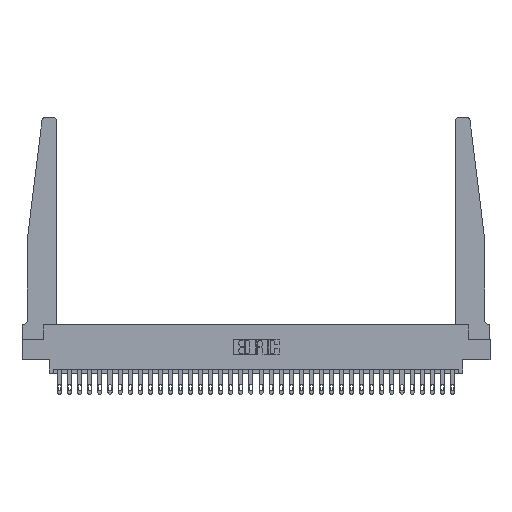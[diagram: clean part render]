
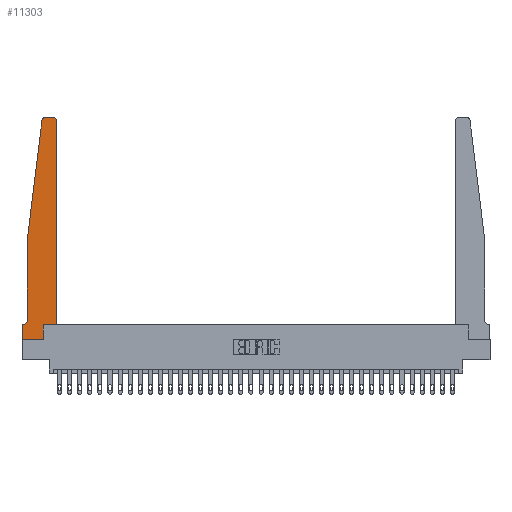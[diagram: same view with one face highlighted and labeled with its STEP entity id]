
A CAD part, top view. The second image highlights one B-rep face of the part: STEP entity #11303.
In plain terms, the highlighted planar face has unit normal (0, 0, 1).
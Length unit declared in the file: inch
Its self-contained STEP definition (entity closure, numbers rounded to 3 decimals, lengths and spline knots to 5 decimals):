
#123 = EDGE_CURVE ( 'NONE', #7158, #9645, #1898, .T. ) ;
#701 = LINE ( 'NONE', #27002, #2936 ) ;
#1346 = VECTOR ( 'NONE', #9634, 39.37008 ) ;
#1495 = VERTEX_POINT ( 'NONE', #11443 ) ;
#1792 = DIRECTION ( 'NONE',  ( -1., 0., 0. ) ) ;
#1898 = CIRCLE ( 'NONE', #8048, 0.03 ) ;
#1957 = EDGE_CURVE ( 'NONE', #8215, #24867, #27347, .T. ) ;
#2652 = FACE_OUTER_BOUND ( 'NONE', #3801, .T. ) ;
#2743 = LINE ( 'NONE', #31608, #1346 ) ;
#2936 = VECTOR ( 'NONE', #10459, 39.37008 ) ;
#3801 = EDGE_LOOP ( 'NONE', ( #6980, #9126, #20658, #7525, #21040, #28961, #9816, #30972, #6041, #6611, #29321, #30277 ) ) ;
#4433 = CARTESIAN_POINT ( 'NONE',  ( 0.065, 1.25, 0.37 ) ) ;
#4460 = AXIS2_PLACEMENT_3D ( 'NONE', #30757, #18735, #13747 ) ;
#4726 = CARTESIAN_POINT ( 'NONE',  ( 0.27653, 2.75, 0.37 ) ) ;
#4732 = VERTEX_POINT ( 'NONE', #18431 ) ;
#5006 = VECTOR ( 'NONE', #24131, 39.37008 ) ;
#5258 = CARTESIAN_POINT ( 'NONE',  ( 0.395, 2.75, 0.37 ) ) ;
#5487 = LINE ( 'NONE', #7716, #8465 ) ;
#5634 = CARTESIAN_POINT ( 'NONE',  ( 0.2605, 0., 0.37 ) ) ;
#6041 = ORIENTED_EDGE ( 'NONE', *, *, #28409, .T. ) ;
#6611 = ORIENTED_EDGE ( 'NONE', *, *, #25620, .T. ) ;
#6639 = CARTESIAN_POINT ( 'NONE',  ( 0.27653, 2.72, 0.37 ) ) ;
#6980 = ORIENTED_EDGE ( 'NONE', *, *, #19520, .T. ) ;
#7150 = CARTESIAN_POINT ( 'NONE',  ( 0., 0.1875, 0.37 ) ) ;
#7158 = VERTEX_POINT ( 'NONE', #28090 ) ;
#7253 = VERTEX_POINT ( 'NONE', #18479 ) ;
#7525 = ORIENTED_EDGE ( 'NONE', *, *, #24186, .T. ) ;
#7612 = CARTESIAN_POINT ( 'NONE',  ( 0.2605, 0.18, 0.37 ) ) ;
#7716 = CARTESIAN_POINT ( 'NONE',  ( 0.425, 0.18, 0.37 ) ) ;
#8041 = CARTESIAN_POINT ( 'NONE',  ( 0.065, 1.25, 0.37 ) ) ;
#8048 = AXIS2_PLACEMENT_3D ( 'NONE', #25898, #28929, #28639 ) ;
#8215 = VERTEX_POINT ( 'NONE', #4726 ) ;
#8465 = VECTOR ( 'NONE', #10102, 39.37008 ) ;
#8737 = CARTESIAN_POINT ( 'NONE',  ( 0.24675, 2.72367, 0.37 ) ) ;
#8828 = CARTESIAN_POINT ( 'NONE',  ( 0.425, 0.18, 0.37 ) ) ;
#8996 = LINE ( 'NONE', #13953, #21807 ) ;
#9024 = AXIS2_PLACEMENT_3D ( 'NONE', #7150, #16941, #9701 ) ;
#9095 = VERTEX_POINT ( 'NONE', #30935 ) ;
#9126 = ORIENTED_EDGE ( 'NONE', *, *, #1957, .T. ) ;
#9484 = EDGE_CURVE ( 'NONE', #15782, #9095, #20843, .T. ) ;
#9634 = DIRECTION ( 'NONE',  ( 0., 1., 0. ) ) ;
#9645 = VERTEX_POINT ( 'NONE', #5258 ) ;
#9696 = LINE ( 'NONE', #4433, #5006 ) ;
#9701 = DIRECTION ( 'NONE',  ( 1., 0., 0. ) ) ;
#9816 = ORIENTED_EDGE ( 'NONE', *, *, #13018, .T. ) ;
#10102 = DIRECTION ( 'NONE',  ( 1., 0., 0. ) ) ;
#10104 = DIRECTION ( 'NONE',  ( 0., -1., 0. ) ) ;
#10192 = EDGE_CURVE ( 'NONE', #4732, #15517, #10587, .T. ) ;
#10459 = DIRECTION ( 'NONE',  ( 0., -1., 0. ) ) ;
#10587 = LINE ( 'NONE', #22473, #27391 ) ;
#11303 = ADVANCED_FACE ( 'NONE', ( #2652 ), #14967, .T. ) ;
#11443 = CARTESIAN_POINT ( 'NONE',  ( 0., 0.1875, 0.37 ) ) ;
#12607 = CARTESIAN_POINT ( 'NONE',  ( 0.065, 0.2375, 0.37 ) ) ;
#12836 = EDGE_CURVE ( 'NONE', #24867, #28902, #9696, .T. ) ;
#12977 = DIRECTION ( 'NONE',  ( 1., 0., 0. ) ) ;
#13018 = EDGE_CURVE ( 'NONE', #1495, #4732, #701, .T. ) ;
#13747 = DIRECTION ( 'NONE',  ( -1., 0., 0. ) ) ;
#13953 = CARTESIAN_POINT ( 'NONE',  ( 0.25, 2.75, 0.37 ) ) ;
#14882 = VERTEX_POINT ( 'NONE', #8828 ) ;
#14967 = PLANE ( 'NONE',  #9024 ) ;
#15517 = VERTEX_POINT ( 'NONE', #5634 ) ;
#15782 = VERTEX_POINT ( 'NONE', #12607 ) ;
#16941 = DIRECTION ( 'NONE',  ( 0., 0., 1. ) ) ;
#18431 = CARTESIAN_POINT ( 'NONE',  ( 0., 0., 0.37 ) ) ;
#18479 = CARTESIAN_POINT ( 'NONE',  ( 0.2605, 0.18, 0.37 ) ) ;
#18735 = DIRECTION ( 'NONE',  ( 0., 0., -1. ) ) ;
#19520 = EDGE_CURVE ( 'NONE', #9645, #8215, #8996, .T. ) ;
#19577 = EDGE_CURVE ( 'NONE', #14882, #7158, #2743, .T. ) ;
#20658 = ORIENTED_EDGE ( 'NONE', *, *, #12836, .T. ) ;
#20843 = CIRCLE ( 'NONE', #4460, 0.05 ) ;
#21040 = ORIENTED_EDGE ( 'NONE', *, *, #9484, .T. ) ;
#21629 = CARTESIAN_POINT ( 'NONE',  ( 0.065, 0.1875, 0.37 ) ) ;
#21807 = VECTOR ( 'NONE', #1792, 39.37008 ) ;
#22458 = EDGE_CURVE ( 'NONE', #9095, #1495, #30781, .T. ) ;
#22473 = CARTESIAN_POINT ( 'NONE',  ( 0., 0., 0.37 ) ) ;
#23467 = DIRECTION ( 'NONE',  ( 0., 0., 1. ) ) ;
#23962 = VECTOR ( 'NONE', #24443, 39.37008 ) ;
#24131 = DIRECTION ( 'NONE',  ( -0.122, -0.992, 0. ) ) ;
#24186 = EDGE_CURVE ( 'NONE', #28902, #15782, #29678, .T. ) ;
#24272 = LINE ( 'NONE', #7612, #23962 ) ;
#24443 = DIRECTION ( 'NONE',  ( 0., 1., 0. ) ) ;
#24867 = VERTEX_POINT ( 'NONE', #8737 ) ;
#25173 = CARTESIAN_POINT ( 'NONE',  ( 0.065, 1.25, 0.37 ) ) ;
#25620 = EDGE_CURVE ( 'NONE', #7253, #14882, #5487, .T. ) ;
#25877 = VECTOR ( 'NONE', #10104, 39.37008 ) ;
#25898 = CARTESIAN_POINT ( 'NONE',  ( 0.395, 2.72, 0.37 ) ) ;
#26173 = DIRECTION ( 'NONE',  ( 1., 0., 0. ) ) ;
#27002 = CARTESIAN_POINT ( 'NONE',  ( 0., 0., 0.37 ) ) ;
#27347 = CIRCLE ( 'NONE', #31451, 0.03 ) ;
#27391 = VECTOR ( 'NONE', #12977, 39.37008 ) ;
#28090 = CARTESIAN_POINT ( 'NONE',  ( 0.425, 2.72, 0.37 ) ) ;
#28409 = EDGE_CURVE ( 'NONE', #15517, #7253, #24272, .T. ) ;
#28538 = DIRECTION ( 'NONE',  ( -1., 0., 0. ) ) ;
#28606 = VECTOR ( 'NONE', #28538, 39.37008 ) ;
#28639 = DIRECTION ( 'NONE',  ( 1., 0., 0. ) ) ;
#28902 = VERTEX_POINT ( 'NONE', #8041 ) ;
#28929 = DIRECTION ( 'NONE',  ( 0., 0., 1. ) ) ;
#28961 = ORIENTED_EDGE ( 'NONE', *, *, #22458, .T. ) ;
#29321 = ORIENTED_EDGE ( 'NONE', *, *, #19577, .T. ) ;
#29678 = LINE ( 'NONE', #25173, #25877 ) ;
#30277 = ORIENTED_EDGE ( 'NONE', *, *, #123, .T. ) ;
#30757 = CARTESIAN_POINT ( 'NONE',  ( 0.015, 0.2375, 0.37 ) ) ;
#30781 = LINE ( 'NONE', #21629, #28606 ) ;
#30935 = CARTESIAN_POINT ( 'NONE',  ( 0.015, 0.1875, 0.37 ) ) ;
#30972 = ORIENTED_EDGE ( 'NONE', *, *, #10192, .T. ) ;
#31451 = AXIS2_PLACEMENT_3D ( 'NONE', #6639, #23467, #26173 ) ;
#31608 = CARTESIAN_POINT ( 'NONE',  ( 0.425, 0.18, 0.37 ) ) ;
